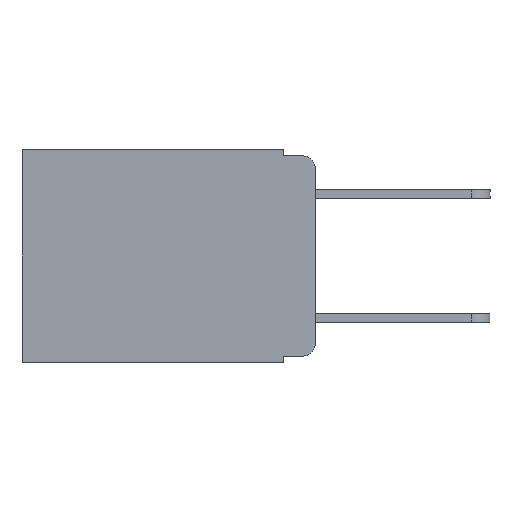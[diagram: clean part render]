
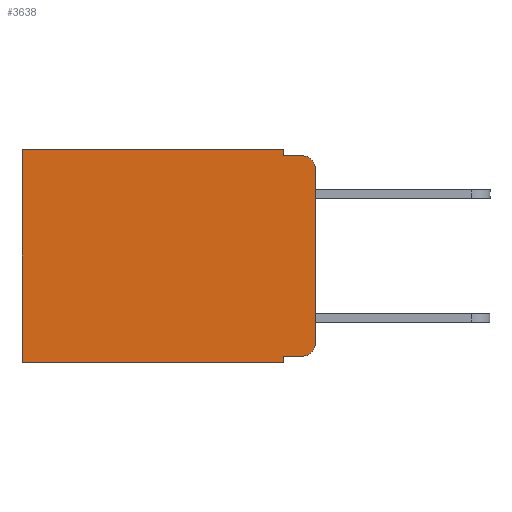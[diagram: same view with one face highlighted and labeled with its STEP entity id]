
A CAD part, left-side view. The second image highlights one B-rep face of the part: STEP entity #3638.
In plain terms, the highlighted planar face has unit normal (-1, 0, 0).
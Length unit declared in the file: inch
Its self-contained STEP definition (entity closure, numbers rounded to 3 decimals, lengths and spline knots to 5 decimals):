
#413 = CARTESIAN_POINT ( 'NONE',  ( 0.298, 0.051, -0.01 ) ) ;
#434 = VERTEX_POINT ( 'NONE', #413 ) ;
#629 = VERTEX_POINT ( 'NONE', #7254 ) ;
#681 = CARTESIAN_POINT ( 'NONE',  ( 0.298, 0., 0. ) ) ;
#688 = CARTESIAN_POINT ( 'NONE',  ( 0.298, 0., -0.343 ) ) ;
#725 = VERTEX_POINT ( 'NONE', #7751 ) ;
#826 = EDGE_CURVE ( 'NONE', #629, #8682, #8946, .T. ) ;
#967 = CARTESIAN_POINT ( 'NONE',  ( 0.298, 0., 0. ) ) ;
#993 = VERTEX_POINT ( 'NONE', #2591 ) ;
#1259 = LINE ( 'NONE', #688, #3399 ) ;
#1263 = CARTESIAN_POINT ( 'NONE',  ( 0.298, 0.473, 0. ) ) ;
#1604 = VERTEX_POINT ( 'NONE', #3998 ) ;
#1612 = VERTEX_POINT ( 'NONE', #6384 ) ;
#2328 = EDGE_CURVE ( 'NONE', #993, #629, #7653, .T. ) ;
#2423 = LINE ( 'NONE', #681, #5162 ) ;
#2443 = CARTESIAN_POINT ( 'NONE',  ( 0.298, 0.473, -0.343 ) ) ;
#2548 = ORIENTED_EDGE ( 'NONE', *, *, #7173, .T. ) ;
#2575 = FACE_OUTER_BOUND ( 'NONE', #5327, .T. ) ;
#2584 = LINE ( 'NONE', #6923, #6405 ) ;
#2591 = CARTESIAN_POINT ( 'NONE',  ( 0.298, 0.051, -0.333 ) ) ;
#2833 = VECTOR ( 'NONE', #9709, 39.37008 ) ;
#2921 = VECTOR ( 'NONE', #8714, 39.37008 ) ;
#2975 = VECTOR ( 'NONE', #8471, 39.37008 ) ;
#3045 = VERTEX_POINT ( 'NONE', #9617 ) ;
#3117 = DIRECTION ( 'NONE',  ( 0., 0., -1. ) ) ;
#3399 = VECTOR ( 'NONE', #3656, 39.37008 ) ;
#3447 = VERTEX_POINT ( 'NONE', #7881 ) ;
#3545 = AXIS2_PLACEMENT_3D ( 'NONE', #9689, #8546, #9707 ) ;
#3638 = ADVANCED_FACE ( 'NONE', ( #2575 ), #4841, .F. ) ;
#3656 = DIRECTION ( 'NONE',  ( 0., 1., 0. ) ) ;
#3741 = CARTESIAN_POINT ( 'NONE',  ( 0.298, 0., 0. ) ) ;
#3791 = CARTESIAN_POINT ( 'NONE',  ( 0.298, 0.02, -0.313 ) ) ;
#3917 = CARTESIAN_POINT ( 'NONE',  ( 0.298, 0., -0.313 ) ) ;
#3998 = CARTESIAN_POINT ( 'NONE',  ( 0.298, 0., -0.03 ) ) ;
#4119 = ORIENTED_EDGE ( 'NONE', *, *, #2328, .T. ) ;
#4364 = ORIENTED_EDGE ( 'NONE', *, *, #6936, .T. ) ;
#4539 = DIRECTION ( 'NONE',  ( 1., 0., 0. ) ) ;
#4554 = AXIS2_PLACEMENT_3D ( 'NONE', #3741, #4539, #4717 ) ;
#4603 = ORIENTED_EDGE ( 'NONE', *, *, #7645, .T. ) ;
#4717 = DIRECTION ( 'NONE',  ( 0., 0., -1. ) ) ;
#4841 = PLANE ( 'NONE',  #4554 ) ;
#5041 = ORIENTED_EDGE ( 'NONE', *, *, #8681, .F. ) ;
#5138 = EDGE_CURVE ( 'NONE', #725, #434, #2584, .T. ) ;
#5147 = LINE ( 'NONE', #1263, #2975 ) ;
#5162 = VECTOR ( 'NONE', #7962, 39.37008 ) ;
#5241 = LINE ( 'NONE', #967, #2833 ) ;
#5327 = EDGE_LOOP ( 'NONE', ( #6825, #4603, #5041, #5445, #2548, #4364, #9570, #8271, #4119, #6370 ) ) ;
#5365 = EDGE_CURVE ( 'NONE', #1604, #8682, #2423, .T. ) ;
#5445 = ORIENTED_EDGE ( 'NONE', *, *, #5138, .F. ) ;
#6006 = EDGE_CURVE ( 'NONE', #3447, #6053, #1259, .T. ) ;
#6053 = VERTEX_POINT ( 'NONE', #2443 ) ;
#6150 = CIRCLE ( 'NONE', #3545, 0.02 ) ;
#6210 = LINE ( 'NONE', #7810, #9609 ) ;
#6370 = ORIENTED_EDGE ( 'NONE', *, *, #826, .T. ) ;
#6384 = CARTESIAN_POINT ( 'NONE',  ( 0.298, 0.473, 0. ) ) ;
#6405 = VECTOR ( 'NONE', #3117, 39.37008 ) ;
#6746 = DIRECTION ( 'NONE',  ( 0., 0., -1. ) ) ;
#6825 = ORIENTED_EDGE ( 'NONE', *, *, #5365, .F. ) ;
#6923 = CARTESIAN_POINT ( 'NONE',  ( 0.298, 0.051, 0. ) ) ;
#6936 = EDGE_CURVE ( 'NONE', #1612, #6053, #5147, .T. ) ;
#7133 = AXIS2_PLACEMENT_3D ( 'NONE', #3791, #8460, #7191 ) ;
#7173 = EDGE_CURVE ( 'NONE', #725, #1612, #5241, .T. ) ;
#7191 = DIRECTION ( 'NONE',  ( 0., 0., -1. ) ) ;
#7192 = CARTESIAN_POINT ( 'NONE',  ( 0.298, 0.051, -0.333 ) ) ;
#7254 = CARTESIAN_POINT ( 'NONE',  ( 0.298, 0.02, -0.333 ) ) ;
#7430 = DIRECTION ( 'NONE',  ( 0., -1., 0. ) ) ;
#7645 = EDGE_CURVE ( 'NONE', #1604, #3045, #6150, .T. ) ;
#7653 = LINE ( 'NONE', #7192, #9228 ) ;
#7751 = CARTESIAN_POINT ( 'NONE',  ( 0.298, 0.051, 0. ) ) ;
#7810 = CARTESIAN_POINT ( 'NONE',  ( 0.298, 0.051, 0. ) ) ;
#7881 = CARTESIAN_POINT ( 'NONE',  ( 0.298, 0.051, -0.343 ) ) ;
#7962 = DIRECTION ( 'NONE',  ( 0., 0., -1. ) ) ;
#8271 = ORIENTED_EDGE ( 'NONE', *, *, #9160, .F. ) ;
#8460 = DIRECTION ( 'NONE',  ( -1., 0., 0. ) ) ;
#8471 = DIRECTION ( 'NONE',  ( 0., 0., -1. ) ) ;
#8546 = DIRECTION ( 'NONE',  ( -1., 0., 0. ) ) ;
#8681 = EDGE_CURVE ( 'NONE', #434, #3045, #8766, .T. ) ;
#8682 = VERTEX_POINT ( 'NONE', #3917 ) ;
#8714 = DIRECTION ( 'NONE',  ( 0., -1., 0. ) ) ;
#8766 = LINE ( 'NONE', #8802, #2921 ) ;
#8802 = CARTESIAN_POINT ( 'NONE',  ( 0.298, 0.051, -0.01 ) ) ;
#8946 = CIRCLE ( 'NONE', #7133, 0.02 ) ;
#9160 = EDGE_CURVE ( 'NONE', #993, #3447, #6210, .T. ) ;
#9228 = VECTOR ( 'NONE', #7430, 39.37008 ) ;
#9570 = ORIENTED_EDGE ( 'NONE', *, *, #6006, .F. ) ;
#9609 = VECTOR ( 'NONE', #6746, 39.37008 ) ;
#9617 = CARTESIAN_POINT ( 'NONE',  ( 0.298, 0.02, -0.01 ) ) ;
#9689 = CARTESIAN_POINT ( 'NONE',  ( 0.298, 0.02, -0.03 ) ) ;
#9707 = DIRECTION ( 'NONE',  ( 0., 0., -1. ) ) ;
#9709 = DIRECTION ( 'NONE',  ( 0., 1., 0. ) ) ;
